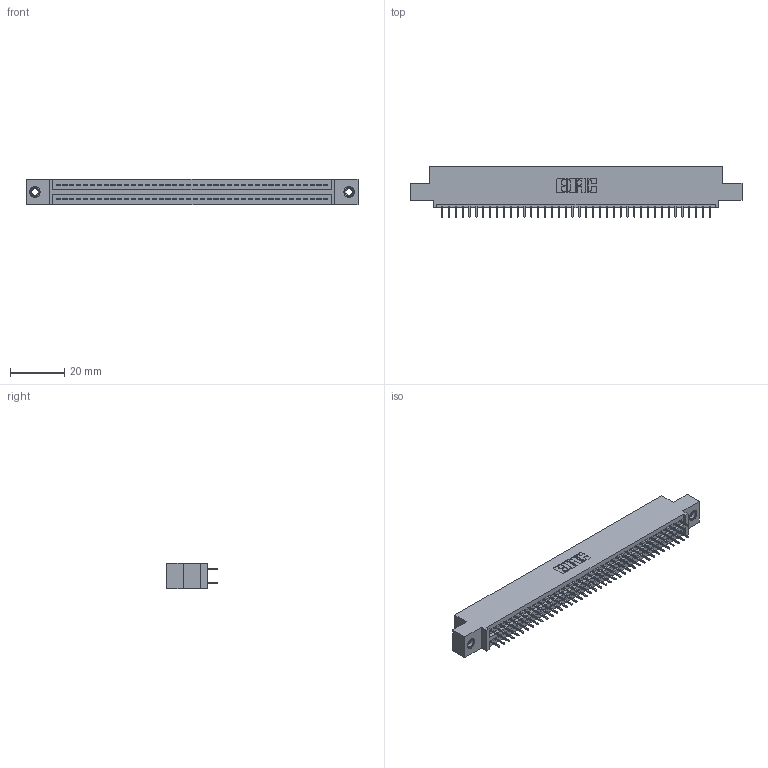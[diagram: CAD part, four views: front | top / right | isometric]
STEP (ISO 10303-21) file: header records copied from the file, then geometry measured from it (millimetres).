
FILE_DESCRIPTION (( 'STEP AP203' ), '1' );
FILE_NAME ('845-080-525-507.STEP', '2020-09-24T01:00:35', ( '' ), ( '' ), 'SwSTEP 2.0', 'SolidWorks 2020', '' );
FILE_SCHEMA (( 'CONFIG_CONTROL_DESIGN' ));
Length unit declared in the file: inch
Products named in the file (4): 845-080-525-507; 345-250-001_345-250-005-103; 345-292-001_345-293-125; 845 Part_0.110 Offset - 0.156 Dia-TI
Assembly tree (83 placements, depth 2):
  845-080-525-507
    845 Part_0.110 Offset - 0.156 Dia-TI
    345-292-001_345-293-125  x80
    345-250-001_345-250-005-103  x2
Bounding box: 122.81 x 18.72 x 9.4 mm (x, y, z)
Volume: 11692.7 mm3; surface area: 16968.9 mm2
Topology: 83 solids, 83 shells, 4510 faces, 12729 edges, 8158 vertices
Faces by surface type: plane 3236, cylinder 1258, cone 12, torus 4
Entity records: 33046 total; most frequent: CARTESIAN_POINT 5523, ORIENTED_EDGE 5450, DIRECTION 4899, EDGE_CURVE 2725, LINE 2417, VECTOR 2417, VERTEX_POINT 1808, AXIS2_PLACEMENT_3D 1241
